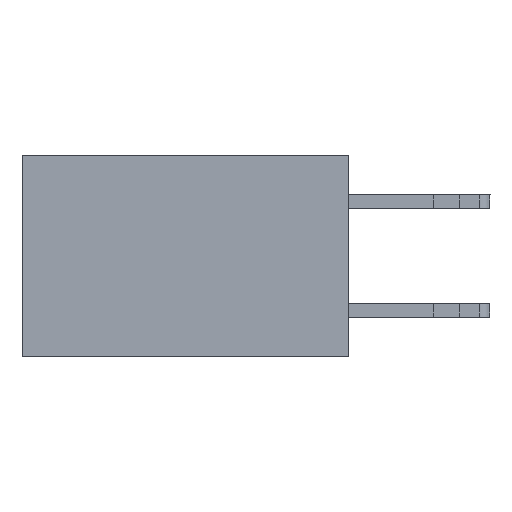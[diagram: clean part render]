
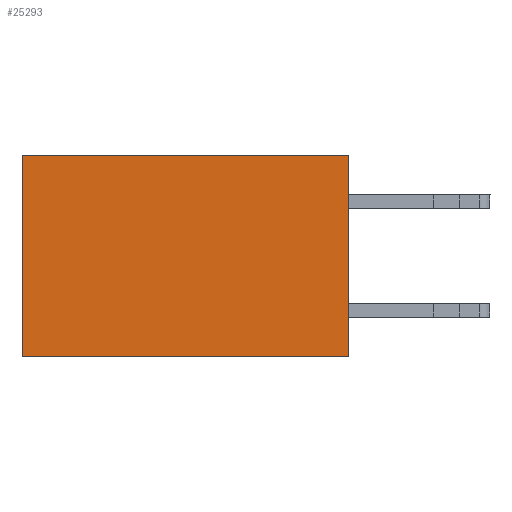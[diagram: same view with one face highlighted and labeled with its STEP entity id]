
A CAD part, left-side view. The second image highlights one B-rep face of the part: STEP entity #25293.
In plain terms, the highlighted planar face has unit normal (-1, 0, 0).
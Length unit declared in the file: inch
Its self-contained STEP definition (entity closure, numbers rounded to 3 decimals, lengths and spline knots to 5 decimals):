
#690 = EDGE_CURVE ( 'NONE', #19816, #16006, #1321, .T. ) ;
#1321 = LINE ( 'NONE', #9235, #25119 ) ;
#2089 = EDGE_CURVE ( 'NONE', #22946, #4912, #7532, .T. ) ;
#2374 = FACE_OUTER_BOUND ( 'NONE', #24243, .T. ) ;
#4912 = VERTEX_POINT ( 'NONE', #20311 ) ;
#4975 = DIRECTION ( 'NONE',  ( 0., 1., 0. ) ) ;
#5011 = LINE ( 'NONE', #12970, #22517 ) ;
#6726 = CARTESIAN_POINT ( 'NONE',  ( 0.298, 0., 0. ) ) ;
#7179 = CARTESIAN_POINT ( 'NONE',  ( 0.298, 0.6, -0.37 ) ) ;
#7532 = LINE ( 'NONE', #23352, #11775 ) ;
#7791 = ORIENTED_EDGE ( 'NONE', *, *, #23699, .T. ) ;
#8346 = ORIENTED_EDGE ( 'NONE', *, *, #690, .F. ) ;
#9235 = CARTESIAN_POINT ( 'NONE',  ( 0.298, 0., -0.37 ) ) ;
#9468 = LINE ( 'NONE', #21363, #18063 ) ;
#10307 = PLANE ( 'NONE',  #16977 ) ;
#11775 = VECTOR ( 'NONE', #19680, 39.37008 ) ;
#12970 = CARTESIAN_POINT ( 'NONE',  ( 0.298, 0.6, 0. ) ) ;
#15112 = DIRECTION ( 'NONE',  ( 0., 0., -1. ) ) ;
#16006 = VERTEX_POINT ( 'NONE', #7179 ) ;
#16414 = DIRECTION ( 'NONE',  ( 1., 0., 0. ) ) ;
#16903 = CARTESIAN_POINT ( 'NONE',  ( 0.298, 0., -0.37 ) ) ;
#16977 = AXIS2_PLACEMENT_3D ( 'NONE', #18255, #16414, #21804 ) ;
#17148 = ORIENTED_EDGE ( 'NONE', *, *, #17681, .F. ) ;
#17681 = EDGE_CURVE ( 'NONE', #22946, #19816, #9468, .T. ) ;
#18063 = VECTOR ( 'NONE', #15112, 39.37008 ) ;
#18255 = CARTESIAN_POINT ( 'NONE',  ( 0.298, 0., 0. ) ) ;
#19680 = DIRECTION ( 'NONE',  ( 0., 1., 0. ) ) ;
#19816 = VERTEX_POINT ( 'NONE', #16903 ) ;
#20311 = CARTESIAN_POINT ( 'NONE',  ( 0.298, 0.6, 0. ) ) ;
#20515 = DIRECTION ( 'NONE',  ( 0., 0., -1. ) ) ;
#20843 = ORIENTED_EDGE ( 'NONE', *, *, #2089, .T. ) ;
#21363 = CARTESIAN_POINT ( 'NONE',  ( 0.298, 0., 0. ) ) ;
#21804 = DIRECTION ( 'NONE',  ( 0., 0., -1. ) ) ;
#22517 = VECTOR ( 'NONE', #20515, 39.37008 ) ;
#22946 = VERTEX_POINT ( 'NONE', #6726 ) ;
#23352 = CARTESIAN_POINT ( 'NONE',  ( 0.298, 0., 0. ) ) ;
#23699 = EDGE_CURVE ( 'NONE', #4912, #16006, #5011, .T. ) ;
#24243 = EDGE_LOOP ( 'NONE', ( #7791, #8346, #17148, #20843 ) ) ;
#25119 = VECTOR ( 'NONE', #4975, 39.37008 ) ;
#25293 = ADVANCED_FACE ( 'NONE', ( #2374 ), #10307, .F. ) ;
